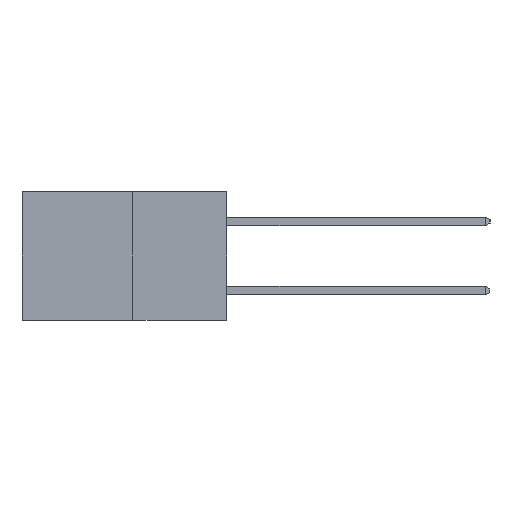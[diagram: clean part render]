
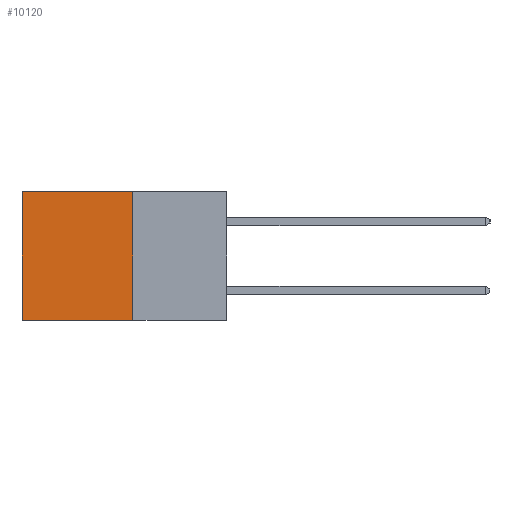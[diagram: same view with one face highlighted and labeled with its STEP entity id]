
A CAD part, left-side view. The second image highlights one B-rep face of the part: STEP entity #10120.
In plain terms, the highlighted planar face has unit normal (-1, 0, 0).
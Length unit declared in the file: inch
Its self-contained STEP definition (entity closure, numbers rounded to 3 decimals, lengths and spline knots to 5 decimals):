
#91 = EDGE_CURVE ( 'NONE', #7041, #14437, #6370, .T. ) ;
#825 = VERTEX_POINT ( 'NONE', #15013 ) ;
#884 = EDGE_LOOP ( 'NONE', ( #4963, #11791, #7791, #15666 ) ) ;
#1122 = VECTOR ( 'NONE', #8173, 39.37008 ) ;
#1305 = CARTESIAN_POINT ( 'NONE',  ( 0.277, 0.27, -0.37 ) ) ;
#1687 = LINE ( 'NONE', #11526, #8243 ) ;
#2056 = VECTOR ( 'NONE', #7951, 39.37008 ) ;
#2671 = DIRECTION ( 'NONE',  ( 0., 0., -1. ) ) ;
#3811 = DIRECTION ( 'NONE',  ( 0., 1., 0. ) ) ;
#3915 = EDGE_CURVE ( 'NONE', #825, #12879, #6077, .T. ) ;
#4624 = EDGE_CURVE ( 'NONE', #12879, #14437, #15718, .T. ) ;
#4963 = ORIENTED_EDGE ( 'NONE', *, *, #91, .T. ) ;
#6077 = LINE ( 'NONE', #14986, #1122 ) ;
#6370 = LINE ( 'NONE', #12938, #2056 ) ;
#7041 = VERTEX_POINT ( 'NONE', #13613 ) ;
#7791 = ORIENTED_EDGE ( 'NONE', *, *, #3915, .F. ) ;
#7847 = PLANE ( 'NONE',  #9152 ) ;
#7951 = DIRECTION ( 'NONE',  ( 0., 0., -1. ) ) ;
#8032 = CARTESIAN_POINT ( 'NONE',  ( 0.277, 0.59, -0.37 ) ) ;
#8173 = DIRECTION ( 'NONE',  ( 0., 0., -1. ) ) ;
#8243 = VECTOR ( 'NONE', #3811, 39.37008 ) ;
#9152 = AXIS2_PLACEMENT_3D ( 'NONE', #1305, #10434, #2671 ) ;
#10020 = DIRECTION ( 'NONE',  ( 0., 1., 0. ) ) ;
#10120 = ADVANCED_FACE ( 'NONE', ( #13430 ), #7847, .F. ) ;
#10434 = DIRECTION ( 'NONE',  ( 1., 0., 0. ) ) ;
#10472 = CARTESIAN_POINT ( 'NONE',  ( 0.277, 0.27, -0.37 ) ) ;
#10707 = EDGE_CURVE ( 'NONE', #825, #7041, #1687, .T. ) ;
#10806 = CARTESIAN_POINT ( 'NONE',  ( 0.277, 0.27, -0.37 ) ) ;
#11526 = CARTESIAN_POINT ( 'NONE',  ( 0.277, 0.27, 0. ) ) ;
#11791 = ORIENTED_EDGE ( 'NONE', *, *, #4624, .F. ) ;
#12043 = VECTOR ( 'NONE', #10020, 39.37008 ) ;
#12879 = VERTEX_POINT ( 'NONE', #10806 ) ;
#12938 = CARTESIAN_POINT ( 'NONE',  ( 0.277, 0.59, -0.37 ) ) ;
#13430 = FACE_OUTER_BOUND ( 'NONE', #884, .T. ) ;
#13613 = CARTESIAN_POINT ( 'NONE',  ( 0.277, 0.59, 0. ) ) ;
#14437 = VERTEX_POINT ( 'NONE', #8032 ) ;
#14986 = CARTESIAN_POINT ( 'NONE',  ( 0.277, 0.27, -0.37 ) ) ;
#15013 = CARTESIAN_POINT ( 'NONE',  ( 0.277, 0.27, 0. ) ) ;
#15666 = ORIENTED_EDGE ( 'NONE', *, *, #10707, .T. ) ;
#15718 = LINE ( 'NONE', #10472, #12043 ) ;
